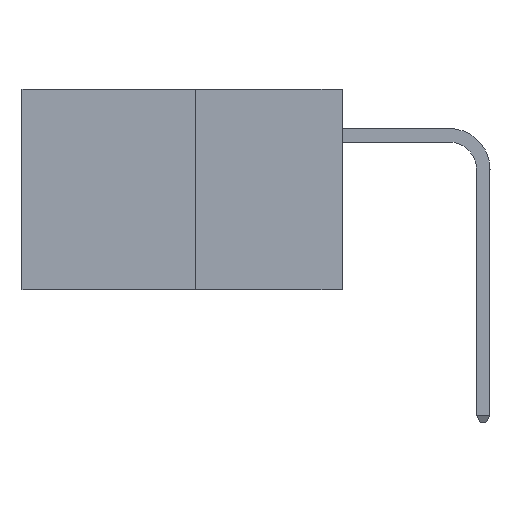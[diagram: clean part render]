
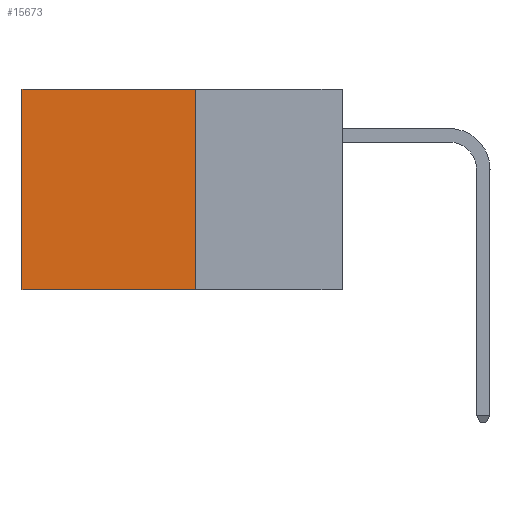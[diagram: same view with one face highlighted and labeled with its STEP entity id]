
A CAD part, left-side view. The second image highlights one B-rep face of the part: STEP entity #15673.
In plain terms, the highlighted planar face has unit normal (-1, 0, 0).
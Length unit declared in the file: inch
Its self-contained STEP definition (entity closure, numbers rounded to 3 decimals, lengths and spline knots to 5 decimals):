
#377 = LINE ( 'NONE', #10547, #15211 ) ;
#2162 = CARTESIAN_POINT ( 'NONE',  ( 0.277, 0.27, 0. ) ) ;
#2415 = DIRECTION ( 'NONE',  ( 0., 0., -1. ) ) ;
#3051 = EDGE_CURVE ( 'NONE', #17725, #22038, #377, .T. ) ;
#4934 = VECTOR ( 'NONE', #16550, 39.37008 ) ;
#5552 = LINE ( 'NONE', #16578, #4934 ) ;
#5891 = FACE_OUTER_BOUND ( 'NONE', #18584, .T. ) ;
#6416 = CARTESIAN_POINT ( 'NONE',  ( 0.277, 0.27, -0.37 ) ) ;
#7027 = PLANE ( 'NONE',  #9315 ) ;
#7089 = ORIENTED_EDGE ( 'NONE', *, *, #21123, .T. ) ;
#7277 = ORIENTED_EDGE ( 'NONE', *, *, #3051, .T. ) ;
#7363 = VERTEX_POINT ( 'NONE', #18613 ) ;
#9315 = AXIS2_PLACEMENT_3D ( 'NONE', #10906, #24099, #12796 ) ;
#9421 = DIRECTION ( 'NONE',  ( 0., 1., 0. ) ) ;
#9527 = ORIENTED_EDGE ( 'NONE', *, *, #9838, .F. ) ;
#9838 = EDGE_CURVE ( 'NONE', #23353, #7363, #5552, .T. ) ;
#10547 = CARTESIAN_POINT ( 'NONE',  ( 0.277, 0.27, 0. ) ) ;
#10906 = CARTESIAN_POINT ( 'NONE',  ( 0.277, 0.27, -0.37 ) ) ;
#12796 = DIRECTION ( 'NONE',  ( 0., 0., -1. ) ) ;
#13722 = ORIENTED_EDGE ( 'NONE', *, *, #24764, .F. ) ;
#14010 = CARTESIAN_POINT ( 'NONE',  ( 0.277, 0.59, -0.37 ) ) ;
#15211 = VECTOR ( 'NONE', #9421, 39.37008 ) ;
#15673 = ADVANCED_FACE ( 'NONE', ( #5891 ), #7027, .F. ) ;
#16101 = VECTOR ( 'NONE', #24122, 39.37008 ) ;
#16539 = CARTESIAN_POINT ( 'NONE',  ( 0.277, 0.59, 0. ) ) ;
#16550 = DIRECTION ( 'NONE',  ( 0., 1., 0. ) ) ;
#16578 = CARTESIAN_POINT ( 'NONE',  ( 0.277, 0.27, -0.37 ) ) ;
#16689 = LINE ( 'NONE', #22263, #16101 ) ;
#17725 = VERTEX_POINT ( 'NONE', #2162 ) ;
#17909 = LINE ( 'NONE', #14010, #22905 ) ;
#18584 = EDGE_LOOP ( 'NONE', ( #7089, #9527, #13722, #7277 ) ) ;
#18613 = CARTESIAN_POINT ( 'NONE',  ( 0.277, 0.59, -0.37 ) ) ;
#21123 = EDGE_CURVE ( 'NONE', #22038, #7363, #17909, .T. ) ;
#22038 = VERTEX_POINT ( 'NONE', #16539 ) ;
#22263 = CARTESIAN_POINT ( 'NONE',  ( 0.277, 0.27, -0.37 ) ) ;
#22905 = VECTOR ( 'NONE', #2415, 39.37008 ) ;
#23353 = VERTEX_POINT ( 'NONE', #6416 ) ;
#24099 = DIRECTION ( 'NONE',  ( 1., 0., 0. ) ) ;
#24122 = DIRECTION ( 'NONE',  ( 0., 0., -1. ) ) ;
#24764 = EDGE_CURVE ( 'NONE', #17725, #23353, #16689, .T. ) ;
